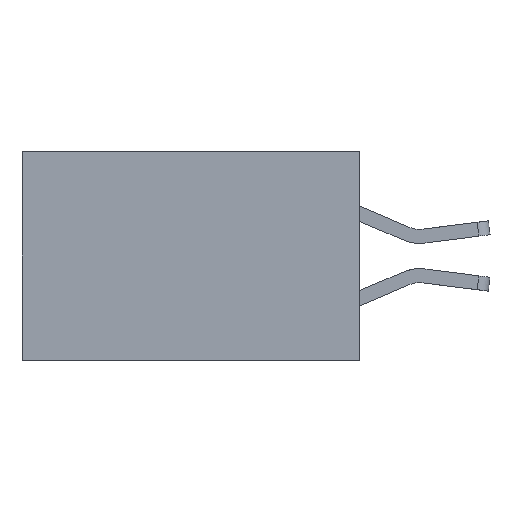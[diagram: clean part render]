
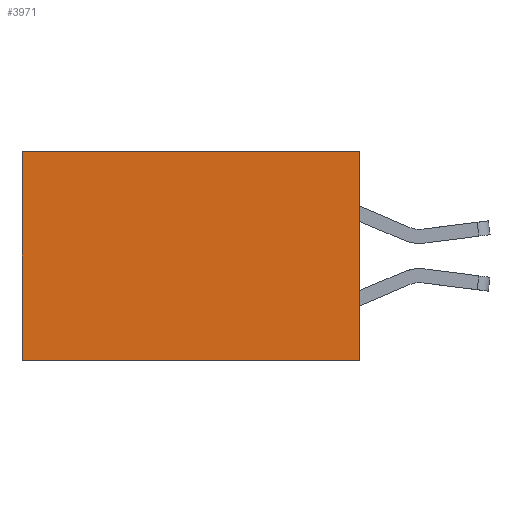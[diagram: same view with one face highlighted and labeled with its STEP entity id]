
A CAD part, left-side view. The second image highlights one B-rep face of the part: STEP entity #3971.
In plain terms, the highlighted planar face has unit normal (-1, 0, 0).
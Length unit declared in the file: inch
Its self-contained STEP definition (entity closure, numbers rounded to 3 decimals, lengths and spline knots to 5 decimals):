
#141 = EDGE_LOOP ( 'NONE', ( #8464, #4732, #8679, #6994 ) ) ;
#284 = EDGE_CURVE ( 'NONE', #6484, #5584, #8860, .T. ) ;
#796 = FACE_OUTER_BOUND ( 'NONE', #141, .T. ) ;
#904 = CARTESIAN_POINT ( 'NONE',  ( 0.2875, 0., -0.37 ) ) ;
#1409 = EDGE_CURVE ( 'NONE', #8169, #5366, #3808, .T. ) ;
#1572 = DIRECTION ( 'NONE',  ( 0., 1., 0. ) ) ;
#2344 = CARTESIAN_POINT ( 'NONE',  ( 0.2875, 0., -0.37 ) ) ;
#2763 = EDGE_CURVE ( 'NONE', #8169, #6484, #9511, .T. ) ;
#3194 = VECTOR ( 'NONE', #1572, 39.37008 ) ;
#3247 = EDGE_CURVE ( 'NONE', #5366, #5584, #9116, .T. ) ;
#3424 = DIRECTION ( 'NONE',  ( 0., 0., -1. ) ) ;
#3778 = CARTESIAN_POINT ( 'NONE',  ( 0.2875, 0., 0. ) ) ;
#3808 = LINE ( 'NONE', #3778, #7655 ) ;
#3971 = ADVANCED_FACE ( 'NONE', ( #796 ), #5808, .F. ) ;
#4159 = CARTESIAN_POINT ( 'NONE',  ( 0.2875, 0.6, 0. ) ) ;
#4226 = CARTESIAN_POINT ( 'NONE',  ( 0.2875, 0., 0. ) ) ;
#4732 = ORIENTED_EDGE ( 'NONE', *, *, #3247, .F. ) ;
#5023 = DIRECTION ( 'NONE',  ( 0., 1., 0. ) ) ;
#5202 = CARTESIAN_POINT ( 'NONE',  ( 0.2875, 0.6, -0.37 ) ) ;
#5366 = VERTEX_POINT ( 'NONE', #904 ) ;
#5584 = VERTEX_POINT ( 'NONE', #5202 ) ;
#5626 = CARTESIAN_POINT ( 'NONE',  ( 0.2875, 0., 0. ) ) ;
#5699 = CARTESIAN_POINT ( 'NONE',  ( 0.2875, 0., 0. ) ) ;
#5808 = PLANE ( 'NONE',  #9166 ) ;
#5825 = CARTESIAN_POINT ( 'NONE',  ( 0.2875, 0.6, 0. ) ) ;
#6086 = DIRECTION ( 'NONE',  ( 0., 0., -1. ) ) ;
#6274 = DIRECTION ( 'NONE',  ( 1., 0., 0. ) ) ;
#6484 = VERTEX_POINT ( 'NONE', #4159 ) ;
#6950 = VECTOR ( 'NONE', #3424, 39.37008 ) ;
#6994 = ORIENTED_EDGE ( 'NONE', *, *, #2763, .T. ) ;
#7030 = VECTOR ( 'NONE', #5023, 39.37008 ) ;
#7655 = VECTOR ( 'NONE', #8979, 39.37008 ) ;
#8169 = VERTEX_POINT ( 'NONE', #4226 ) ;
#8464 = ORIENTED_EDGE ( 'NONE', *, *, #284, .T. ) ;
#8679 = ORIENTED_EDGE ( 'NONE', *, *, #1409, .F. ) ;
#8860 = LINE ( 'NONE', #5825, #6950 ) ;
#8979 = DIRECTION ( 'NONE',  ( 0., 0., -1. ) ) ;
#9116 = LINE ( 'NONE', #2344, #3194 ) ;
#9166 = AXIS2_PLACEMENT_3D ( 'NONE', #5699, #6274, #6086 ) ;
#9511 = LINE ( 'NONE', #5626, #7030 ) ;
